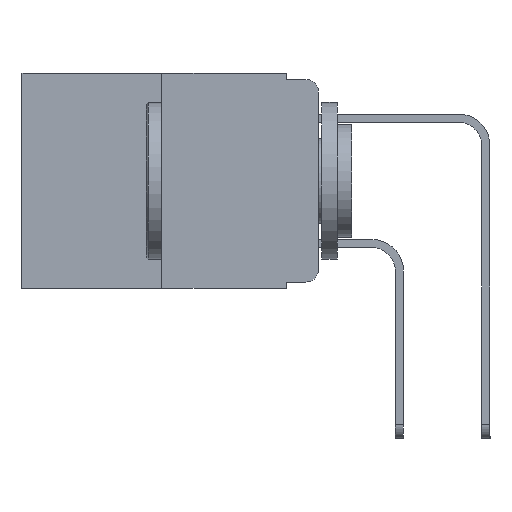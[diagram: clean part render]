
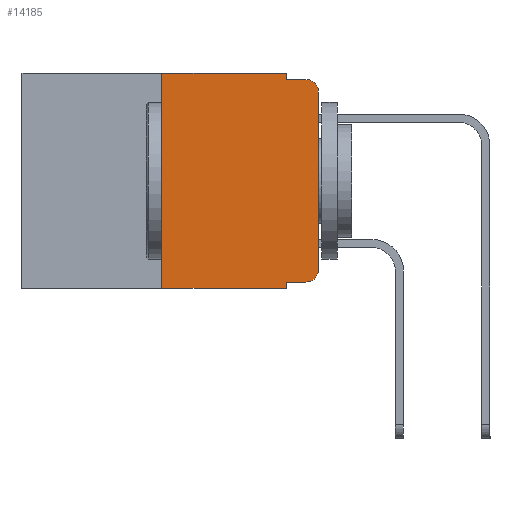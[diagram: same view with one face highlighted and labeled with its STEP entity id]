
A CAD part, left-side view. The second image highlights one B-rep face of the part: STEP entity #14185.
In plain terms, the highlighted planar face has unit normal (-1, 0, 0).
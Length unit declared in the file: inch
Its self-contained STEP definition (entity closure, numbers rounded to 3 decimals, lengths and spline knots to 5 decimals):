
#343 = DIRECTION ( 'NONE',  ( 0., 0., -1. ) ) ;
#567 = EDGE_CURVE ( 'NONE', #1449, #23341, #16749, .T. ) ;
#594 = VERTEX_POINT ( 'NONE', #21156 ) ;
#746 = ORIENTED_EDGE ( 'NONE', *, *, #23483, .T. ) ;
#908 = AXIS2_PLACEMENT_3D ( 'NONE', #12439, #26976, #14544 ) ;
#1132 = CARTESIAN_POINT ( 'NONE',  ( 0., 0.02, -0.01 ) ) ;
#1269 = ORIENTED_EDGE ( 'NONE', *, *, #5912, .F. ) ;
#1449 = VERTEX_POINT ( 'NONE', #24918 ) ;
#1862 = ORIENTED_EDGE ( 'NONE', *, *, #11239, .T. ) ;
#2090 = CARTESIAN_POINT ( 'NONE',  ( 0., 0.02, -0.313 ) ) ;
#2369 = LINE ( 'NONE', #8551, #24672 ) ;
#2451 = ORIENTED_EDGE ( 'NONE', *, *, #4118, .T. ) ;
#2498 = CARTESIAN_POINT ( 'NONE',  ( 0., 0.051, -0.333 ) ) ;
#2795 = ORIENTED_EDGE ( 'NONE', *, *, #9477, .T. ) ;
#3728 = CARTESIAN_POINT ( 'NONE',  ( 0., 0.051, 0. ) ) ;
#4118 = EDGE_CURVE ( 'NONE', #9560, #24508, #24130, .T. ) ;
#4225 = DIRECTION ( 'NONE',  ( 0., 0., -1. ) ) ;
#4248 = VERTEX_POINT ( 'NONE', #23391 ) ;
#4596 = VECTOR ( 'NONE', #14327, 39.37008 ) ;
#4783 = ORIENTED_EDGE ( 'NONE', *, *, #25046, .F. ) ;
#4862 = EDGE_CURVE ( 'NONE', #4248, #15186, #17567, .T. ) ;
#4896 = VECTOR ( 'NONE', #343, 39.37008 ) ;
#5387 = VECTOR ( 'NONE', #8790, 39.37008 ) ;
#5440 = ORIENTED_EDGE ( 'NONE', *, *, #567, .F. ) ;
#5912 = EDGE_CURVE ( 'NONE', #10380, #19550, #12879, .T. ) ;
#6671 = CARTESIAN_POINT ( 'NONE',  ( 0., 0.051, 0. ) ) ;
#7233 = VECTOR ( 'NONE', #24015, 39.37008 ) ;
#7430 = ORIENTED_EDGE ( 'NONE', *, *, #18573, .F. ) ;
#7696 = FACE_OUTER_BOUND ( 'NONE', #17791, .T. ) ;
#8267 = CARTESIAN_POINT ( 'NONE',  ( 0., 0.473, -0.343 ) ) ;
#8551 = CARTESIAN_POINT ( 'NONE',  ( 0., 0., 0. ) ) ;
#8790 = DIRECTION ( 'NONE',  ( 0., -1., 0. ) ) ;
#9477 = EDGE_CURVE ( 'NONE', #594, #15186, #9809, .T. ) ;
#9560 = VERTEX_POINT ( 'NONE', #21009 ) ;
#9809 = CIRCLE ( 'NONE', #908, 0.02 ) ;
#10380 = VERTEX_POINT ( 'NONE', #20751 ) ;
#10554 = LINE ( 'NONE', #6671, #4896 ) ;
#11172 = VECTOR ( 'NONE', #13558, 39.37008 ) ;
#11239 = EDGE_CURVE ( 'NONE', #10380, #9560, #18552, .T. ) ;
#12232 = CARTESIAN_POINT ( 'NONE',  ( 0., 0.25, 0. ) ) ;
#12439 = CARTESIAN_POINT ( 'NONE',  ( 0., 0.02, -0.03 ) ) ;
#12879 = LINE ( 'NONE', #17738, #7233 ) ;
#12915 = AXIS2_PLACEMENT_3D ( 'NONE', #18009, #26360, #13917 ) ;
#13195 = EDGE_CURVE ( 'NONE', #24961, #19550, #26374, .T. ) ;
#13265 = AXIS2_PLACEMENT_3D ( 'NONE', #2090, #16853, #4225 ) ;
#13558 = DIRECTION ( 'NONE',  ( 0., -1., 0. ) ) ;
#13619 = CARTESIAN_POINT ( 'NONE',  ( 0., 0.473, 0. ) ) ;
#13831 = PLANE ( 'NONE',  #12915 ) ;
#13917 = DIRECTION ( 'NONE',  ( 0., 0., -1. ) ) ;
#14185 = ADVANCED_FACE ( 'NONE', ( #7696 ), #13831, .F. ) ;
#14327 = DIRECTION ( 'NONE',  ( 0., 0., 1. ) ) ;
#14544 = DIRECTION ( 'NONE',  ( 0., 0., -1. ) ) ;
#15186 = VERTEX_POINT ( 'NONE', #1132 ) ;
#16647 = VECTOR ( 'NONE', #22900, 39.37008 ) ;
#16749 = LINE ( 'NONE', #13619, #11172 ) ;
#16830 = CARTESIAN_POINT ( 'NONE',  ( 0., 0.25, -0.343 ) ) ;
#16853 = DIRECTION ( 'NONE',  ( -1., 0., 0. ) ) ;
#16942 = VECTOR ( 'NONE', #19876, 39.37008 ) ;
#17567 = LINE ( 'NONE', #17800, #16942 ) ;
#17738 = CARTESIAN_POINT ( 'NONE',  ( 0., 0.051, 0. ) ) ;
#17791 = EDGE_LOOP ( 'NONE', ( #746, #2795, #19544, #4783, #5440, #7430, #18603, #1269, #1862, #2451 ) ) ;
#17800 = CARTESIAN_POINT ( 'NONE',  ( 0., 0.051, -0.01 ) ) ;
#18009 = CARTESIAN_POINT ( 'NONE',  ( 0., 0.473, 0. ) ) ;
#18552 = LINE ( 'NONE', #2498, #5387 ) ;
#18573 = EDGE_CURVE ( 'NONE', #24961, #1449, #22008, .T. ) ;
#18603 = ORIENTED_EDGE ( 'NONE', *, *, #13195, .T. ) ;
#19544 = ORIENTED_EDGE ( 'NONE', *, *, #4862, .F. ) ;
#19550 = VERTEX_POINT ( 'NONE', #21845 ) ;
#19876 = DIRECTION ( 'NONE',  ( 0., -1., 0. ) ) ;
#20751 = CARTESIAN_POINT ( 'NONE',  ( 0., 0.051, -0.333 ) ) ;
#21009 = CARTESIAN_POINT ( 'NONE',  ( 0., 0.02, -0.333 ) ) ;
#21105 = DIRECTION ( 'NONE',  ( 0., 0., 1. ) ) ;
#21156 = CARTESIAN_POINT ( 'NONE',  ( 0., 0., -0.03 ) ) ;
#21845 = CARTESIAN_POINT ( 'NONE',  ( 0., 0.051, -0.343 ) ) ;
#22008 = LINE ( 'NONE', #12232, #4596 ) ;
#22900 = DIRECTION ( 'NONE',  ( 0., -1., 0. ) ) ;
#23341 = VERTEX_POINT ( 'NONE', #3728 ) ;
#23391 = CARTESIAN_POINT ( 'NONE',  ( 0., 0.051, -0.01 ) ) ;
#23483 = EDGE_CURVE ( 'NONE', #24508, #594, #2369, .T. ) ;
#24015 = DIRECTION ( 'NONE',  ( 0., 0., -1. ) ) ;
#24130 = CIRCLE ( 'NONE', #13265, 0.02 ) ;
#24508 = VERTEX_POINT ( 'NONE', #26364 ) ;
#24672 = VECTOR ( 'NONE', #21105, 39.37008 ) ;
#24918 = CARTESIAN_POINT ( 'NONE',  ( 0., 0.25, 0. ) ) ;
#24961 = VERTEX_POINT ( 'NONE', #16830 ) ;
#25046 = EDGE_CURVE ( 'NONE', #23341, #4248, #10554, .T. ) ;
#26360 = DIRECTION ( 'NONE',  ( 1., 0., 0. ) ) ;
#26364 = CARTESIAN_POINT ( 'NONE',  ( 0., 0., -0.313 ) ) ;
#26374 = LINE ( 'NONE', #8267, #16647 ) ;
#26976 = DIRECTION ( 'NONE',  ( -1., 0., 0. ) ) ;
